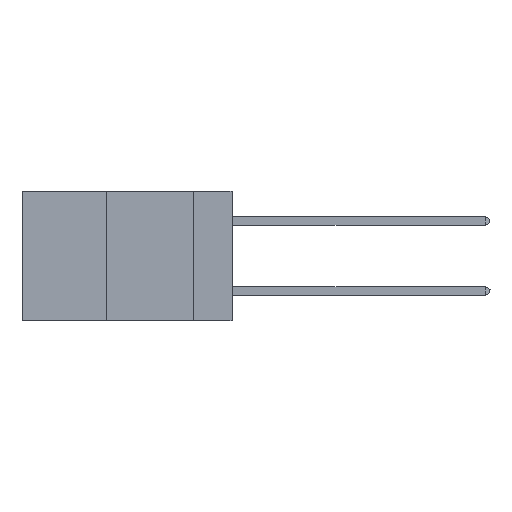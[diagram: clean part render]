
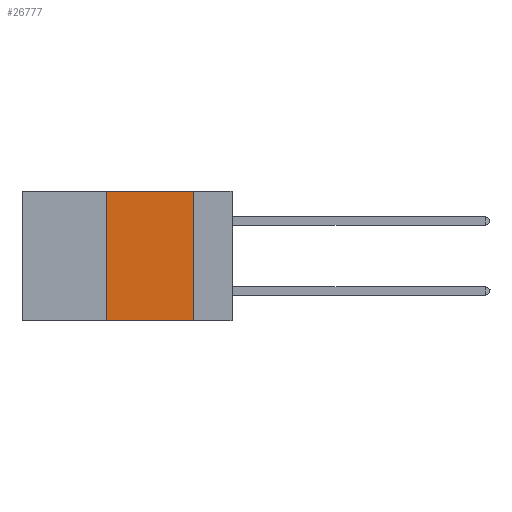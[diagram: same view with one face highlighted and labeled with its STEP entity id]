
A CAD part, left-side view. The second image highlights one B-rep face of the part: STEP entity #26777.
In plain terms, the highlighted planar face has unit normal (-1, 0, 0).
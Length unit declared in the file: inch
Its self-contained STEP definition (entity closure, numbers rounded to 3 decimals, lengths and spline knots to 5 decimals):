
#1 = EDGE_CURVE ( 'NONE', #21700, #19964, #18171, .T. ) ;
#1430 = ORIENTED_EDGE ( 'NONE', *, *, #2785, .T. ) ;
#2785 = EDGE_CURVE ( 'NONE', #21700, #9461, #9851, .T. ) ;
#3221 = ORIENTED_EDGE ( 'NONE', *, *, #21181, .F. ) ;
#4160 = PLANE ( 'NONE',  #7224 ) ;
#4297 = LINE ( 'NONE', #15420, #6836 ) ;
#5210 = VECTOR ( 'NONE', #14614, 39.37008 ) ;
#6836 = VECTOR ( 'NONE', #27041, 39.37008 ) ;
#7224 = AXIS2_PLACEMENT_3D ( 'NONE', #26005, #22951, #34009 ) ;
#9391 = CARTESIAN_POINT ( 'NONE',  ( 0., 0.11, 0. ) ) ;
#9461 = VERTEX_POINT ( 'NONE', #27922 ) ;
#9484 = ORIENTED_EDGE ( 'NONE', *, *, #11270, .F. ) ;
#9851 = LINE ( 'NONE', #20967, #10509 ) ;
#10509 = VECTOR ( 'NONE', #28950, 39.37008 ) ;
#11270 = EDGE_CURVE ( 'NONE', #19964, #12556, #17354, .T. ) ;
#12517 = CARTESIAN_POINT ( 'NONE',  ( 0., 0.36, 0. ) ) ;
#12556 = VERTEX_POINT ( 'NONE', #9391 ) ;
#13469 = ORIENTED_EDGE ( 'NONE', *, *, #1, .F. ) ;
#14119 = CARTESIAN_POINT ( 'NONE',  ( 0., 0.36, -0.37 ) ) ;
#14614 = DIRECTION ( 'NONE',  ( 0., -1., 0. ) ) ;
#15420 = CARTESIAN_POINT ( 'NONE',  ( 0., 0.11, 0. ) ) ;
#17354 = LINE ( 'NONE', #28433, #5210 ) ;
#18171 = LINE ( 'NONE', #12517, #31072 ) ;
#19964 = VERTEX_POINT ( 'NONE', #27209 ) ;
#20967 = CARTESIAN_POINT ( 'NONE',  ( 0., 0.6, -0.37 ) ) ;
#21181 = EDGE_CURVE ( 'NONE', #12556, #9461, #4297, .T. ) ;
#21700 = VERTEX_POINT ( 'NONE', #14119 ) ;
#22951 = DIRECTION ( 'NONE',  ( 1., 0., 0. ) ) ;
#25842 = FACE_OUTER_BOUND ( 'NONE', #29820, .T. ) ;
#26005 = CARTESIAN_POINT ( 'NONE',  ( 0., 0.6, 0. ) ) ;
#26777 = ADVANCED_FACE ( 'NONE', ( #25842 ), #4160, .F. ) ;
#27041 = DIRECTION ( 'NONE',  ( 0., 0., -1. ) ) ;
#27209 = CARTESIAN_POINT ( 'NONE',  ( 0., 0.36, 0. ) ) ;
#27922 = CARTESIAN_POINT ( 'NONE',  ( 0., 0.11, -0.37 ) ) ;
#28433 = CARTESIAN_POINT ( 'NONE',  ( 0., 0.6, 0. ) ) ;
#28950 = DIRECTION ( 'NONE',  ( 0., -1., 0. ) ) ;
#29820 = EDGE_LOOP ( 'NONE', ( #3221, #9484, #13469, #1430 ) ) ;
#31072 = VECTOR ( 'NONE', #31953, 39.37008 ) ;
#31953 = DIRECTION ( 'NONE',  ( 0., 0., 1. ) ) ;
#34009 = DIRECTION ( 'NONE',  ( 0., 0., -1. ) ) ;
